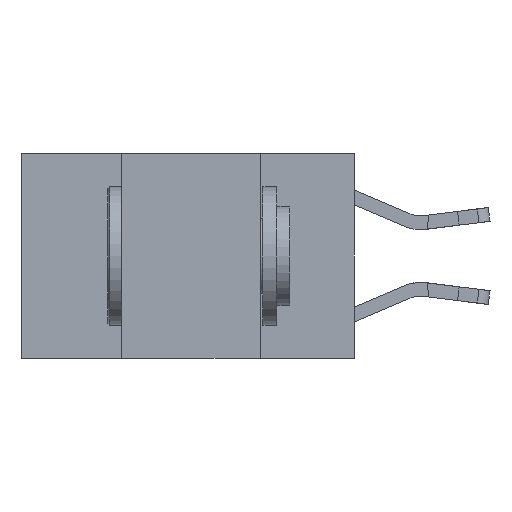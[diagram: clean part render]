
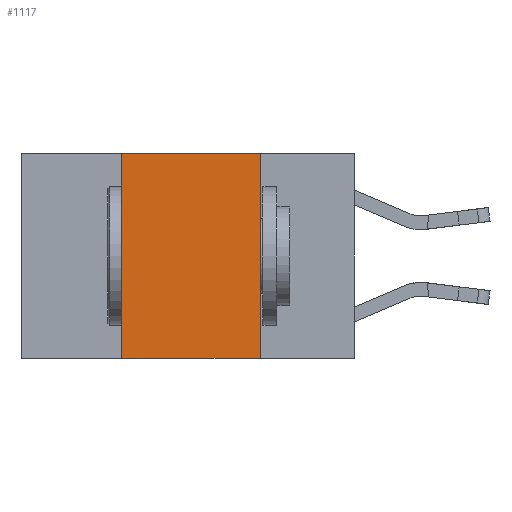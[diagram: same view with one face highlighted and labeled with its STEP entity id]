
A CAD part, left-side view. The second image highlights one B-rep face of the part: STEP entity #1117.
In plain terms, the highlighted planar face has unit normal (-1, 0, 0).
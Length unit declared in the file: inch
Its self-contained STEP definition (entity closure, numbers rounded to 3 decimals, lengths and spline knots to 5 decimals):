
#1117 = ADVANCED_FACE ( 'NONE', ( #6065 ), #11606, .F. ) ;
#1325 = CARTESIAN_POINT ( 'NONE',  ( 0., 0.42, 0. ) ) ;
#2534 = VECTOR ( 'NONE', #6750, 39.37008 ) ;
#3829 = VECTOR ( 'NONE', #17454, 39.37008 ) ;
#4108 = AXIS2_PLACEMENT_3D ( 'NONE', #8035, #13316, #6189 ) ;
#4288 = VERTEX_POINT ( 'NONE', #19919 ) ;
#4423 = LINE ( 'NONE', #14018, #2534 ) ;
#6065 = FACE_OUTER_BOUND ( 'NONE', #15683, .T. ) ;
#6189 = DIRECTION ( 'NONE',  ( 0., 0., -1. ) ) ;
#6723 = ORIENTED_EDGE ( 'NONE', *, *, #16158, .F. ) ;
#6750 = DIRECTION ( 'NONE',  ( 0., -1., 0. ) ) ;
#8035 = CARTESIAN_POINT ( 'NONE',  ( 0., 0.6, 0. ) ) ;
#8334 = LINE ( 'NONE', #15606, #3829 ) ;
#9955 = ORIENTED_EDGE ( 'NONE', *, *, #13574, .F. ) ;
#10014 = CARTESIAN_POINT ( 'NONE',  ( 0., 0.42, -0.37 ) ) ;
#10293 = CARTESIAN_POINT ( 'NONE',  ( 0., 0.17, 0. ) ) ;
#10660 = LINE ( 'NONE', #1325, #22688 ) ;
#11606 = PLANE ( 'NONE',  #4108 ) ;
#13129 = EDGE_CURVE ( 'NONE', #22700, #14674, #4423, .T. ) ;
#13316 = DIRECTION ( 'NONE',  ( 1., 0., 0. ) ) ;
#13574 = EDGE_CURVE ( 'NONE', #18760, #14674, #21253, .T. ) ;
#13851 = DIRECTION ( 'NONE',  ( 0., 0., -1. ) ) ;
#14018 = CARTESIAN_POINT ( 'NONE',  ( 0., 0.6, -0.37 ) ) ;
#14188 = CARTESIAN_POINT ( 'NONE',  ( 0., 0.17, 0. ) ) ;
#14674 = VERTEX_POINT ( 'NONE', #23995 ) ;
#15606 = CARTESIAN_POINT ( 'NONE',  ( 0., 0.6, 0. ) ) ;
#15683 = EDGE_LOOP ( 'NONE', ( #9955, #6723, #16646, #23162 ) ) ;
#16158 = EDGE_CURVE ( 'NONE', #4288, #18760, #8334, .T. ) ;
#16203 = EDGE_CURVE ( 'NONE', #22700, #4288, #10660, .T. ) ;
#16646 = ORIENTED_EDGE ( 'NONE', *, *, #16203, .F. ) ;
#17454 = DIRECTION ( 'NONE',  ( 0., -1., 0. ) ) ;
#18303 = DIRECTION ( 'NONE',  ( 0., 0., 1. ) ) ;
#18760 = VERTEX_POINT ( 'NONE', #14188 ) ;
#19919 = CARTESIAN_POINT ( 'NONE',  ( 0., 0.42, 0. ) ) ;
#21253 = LINE ( 'NONE', #10293, #23762 ) ;
#22688 = VECTOR ( 'NONE', #18303, 39.37008 ) ;
#22700 = VERTEX_POINT ( 'NONE', #10014 ) ;
#23162 = ORIENTED_EDGE ( 'NONE', *, *, #13129, .T. ) ;
#23762 = VECTOR ( 'NONE', #13851, 39.37008 ) ;
#23995 = CARTESIAN_POINT ( 'NONE',  ( 0., 0.17, -0.37 ) ) ;
